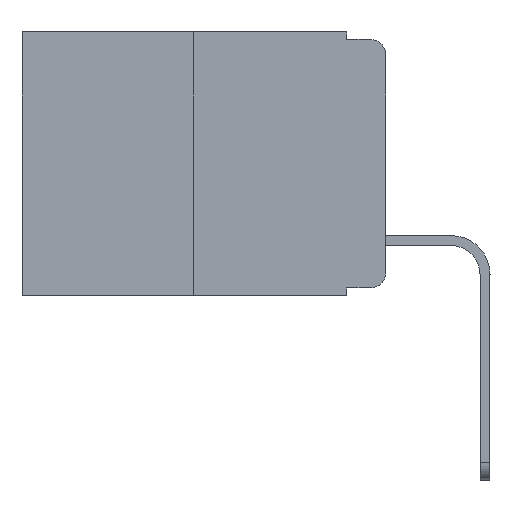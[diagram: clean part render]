
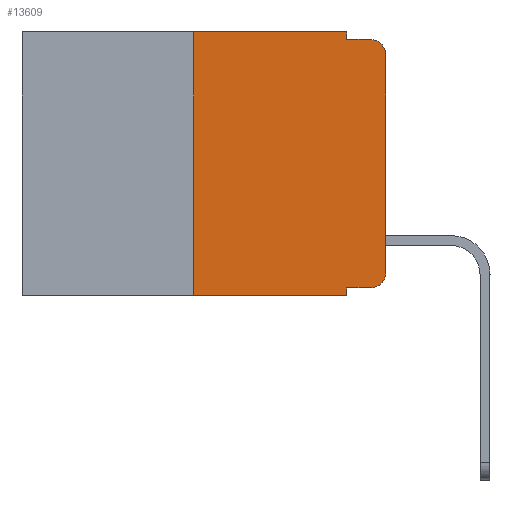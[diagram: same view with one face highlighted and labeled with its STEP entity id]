
A CAD part, left-side view. The second image highlights one B-rep face of the part: STEP entity #13609.
In plain terms, the highlighted planar face has unit normal (-1, 0, 0).
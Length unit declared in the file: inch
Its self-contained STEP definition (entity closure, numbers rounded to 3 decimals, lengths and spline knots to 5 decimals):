
#47 = CARTESIAN_POINT ( 'NONE',  ( 0., 0.25, -0.343 ) ) ;
#64 = CARTESIAN_POINT ( 'NONE',  ( 0., 0.051, 0. ) ) ;
#409 = DIRECTION ( 'NONE',  ( 0., 0., -1. ) ) ;
#425 = CARTESIAN_POINT ( 'NONE',  ( 0., 0., -0.313 ) ) ;
#571 = CARTESIAN_POINT ( 'NONE',  ( 0., 0.051, 0. ) ) ;
#805 = ORIENTED_EDGE ( 'NONE', *, *, #11514, .F. ) ;
#902 = ORIENTED_EDGE ( 'NONE', *, *, #3886, .F. ) ;
#1090 = VECTOR ( 'NONE', #4679, 39.37008 ) ;
#1252 = CARTESIAN_POINT ( 'NONE',  ( 0., 0.473, -0.343 ) ) ;
#1326 = DIRECTION ( 'NONE',  ( -1., 0., 0. ) ) ;
#1520 = EDGE_CURVE ( 'NONE', #8111, #6026, #4271, .T. ) ;
#1595 = EDGE_CURVE ( 'NONE', #8111, #5407, #14626, .T. ) ;
#1687 = VERTEX_POINT ( 'NONE', #5878 ) ;
#1738 = EDGE_CURVE ( 'NONE', #6319, #5173, #14802, .T. ) ;
#2243 = EDGE_CURVE ( 'NONE', #6086, #14339, #12147, .T. ) ;
#2329 = PLANE ( 'NONE',  #9129 ) ;
#3164 = CARTESIAN_POINT ( 'NONE',  ( 0., 0.02, -0.333 ) ) ;
#3420 = EDGE_CURVE ( 'NONE', #1687, #6319, #4641, .T. ) ;
#3616 = DIRECTION ( 'NONE',  ( 0., 0., -1. ) ) ;
#3622 = VERTEX_POINT ( 'NONE', #12099 ) ;
#3840 = EDGE_CURVE ( 'NONE', #3622, #13777, #6791, .T. ) ;
#3886 = EDGE_CURVE ( 'NONE', #1687, #6026, #6254, .T. ) ;
#4117 = ORIENTED_EDGE ( 'NONE', *, *, #14373, .T. ) ;
#4271 = LINE ( 'NONE', #1252, #13584 ) ;
#4641 = LINE ( 'NONE', #10659, #7683 ) ;
#4679 = DIRECTION ( 'NONE',  ( 0., -1., 0. ) ) ;
#5173 = VERTEX_POINT ( 'NONE', #425 ) ;
#5222 = CARTESIAN_POINT ( 'NONE',  ( 0., 0., 0. ) ) ;
#5407 = VERTEX_POINT ( 'NONE', #14429 ) ;
#5878 = CARTESIAN_POINT ( 'NONE',  ( 0., 0.051, -0.333 ) ) ;
#5891 = VECTOR ( 'NONE', #8561, 39.37008 ) ;
#6026 = VERTEX_POINT ( 'NONE', #13424 ) ;
#6086 = VERTEX_POINT ( 'NONE', #7729 ) ;
#6179 = EDGE_LOOP ( 'NONE', ( #4117, #11406, #805, #11504, #7063, #6339, #13868, #902, #12164, #9971 ) ) ;
#6184 = VECTOR ( 'NONE', #10897, 39.37008 ) ;
#6254 = LINE ( 'NONE', #64, #6424 ) ;
#6319 = VERTEX_POINT ( 'NONE', #3164 ) ;
#6339 = ORIENTED_EDGE ( 'NONE', *, *, #1595, .F. ) ;
#6424 = VECTOR ( 'NONE', #8051, 39.37008 ) ;
#6791 = CIRCLE ( 'NONE', #14113, 0.02 ) ;
#7063 = ORIENTED_EDGE ( 'NONE', *, *, #10193, .F. ) ;
#7683 = VECTOR ( 'NONE', #10703, 39.37008 ) ;
#7729 = CARTESIAN_POINT ( 'NONE',  ( 0., 0.051, 0. ) ) ;
#8051 = DIRECTION ( 'NONE',  ( 0., 0., -1. ) ) ;
#8089 = CARTESIAN_POINT ( 'NONE',  ( 0., 0.473, 0. ) ) ;
#8111 = VERTEX_POINT ( 'NONE', #47 ) ;
#8250 = DIRECTION ( 'NONE',  ( 0., 0., -1. ) ) ;
#8561 = DIRECTION ( 'NONE',  ( 0., 0., -1. ) ) ;
#8996 = LINE ( 'NONE', #11500, #1090 ) ;
#9129 = AXIS2_PLACEMENT_3D ( 'NONE', #8089, #9260, #3616 ) ;
#9260 = DIRECTION ( 'NONE',  ( 1., 0., 0. ) ) ;
#9635 = CARTESIAN_POINT ( 'NONE',  ( 0., 0.02, -0.01 ) ) ;
#9728 = AXIS2_PLACEMENT_3D ( 'NONE', #11967, #1326, #409 ) ;
#9971 = ORIENTED_EDGE ( 'NONE', *, *, #1738, .T. ) ;
#10193 = EDGE_CURVE ( 'NONE', #5407, #6086, #8996, .T. ) ;
#10221 = DIRECTION ( 'NONE',  ( 0., -1., 0. ) ) ;
#10350 = DIRECTION ( 'NONE',  ( -1., 0., 0. ) ) ;
#10493 = CARTESIAN_POINT ( 'NONE',  ( 0., 0.02, -0.03 ) ) ;
#10528 = DIRECTION ( 'NONE',  ( 0., 0., 1. ) ) ;
#10538 = VECTOR ( 'NONE', #10528, 39.37008 ) ;
#10659 = CARTESIAN_POINT ( 'NONE',  ( 0., 0.051, -0.333 ) ) ;
#10668 = LINE ( 'NONE', #5222, #6184 ) ;
#10703 = DIRECTION ( 'NONE',  ( 0., -1., 0. ) ) ;
#10709 = CARTESIAN_POINT ( 'NONE',  ( 0., 0.051, -0.01 ) ) ;
#10897 = DIRECTION ( 'NONE',  ( 0., 0., 1. ) ) ;
#11219 = FACE_OUTER_BOUND ( 'NONE', #6179, .T. ) ;
#11406 = ORIENTED_EDGE ( 'NONE', *, *, #3840, .T. ) ;
#11500 = CARTESIAN_POINT ( 'NONE',  ( 0., 0.473, 0. ) ) ;
#11504 = ORIENTED_EDGE ( 'NONE', *, *, #2243, .F. ) ;
#11514 = EDGE_CURVE ( 'NONE', #14339, #13777, #11787, .T. ) ;
#11787 = LINE ( 'NONE', #10709, #11974 ) ;
#11853 = DIRECTION ( 'NONE',  ( 0., -1., 0. ) ) ;
#11967 = CARTESIAN_POINT ( 'NONE',  ( 0., 0.02, -0.313 ) ) ;
#11974 = VECTOR ( 'NONE', #11853, 39.37008 ) ;
#12099 = CARTESIAN_POINT ( 'NONE',  ( 0., 0., -0.03 ) ) ;
#12147 = LINE ( 'NONE', #571, #5891 ) ;
#12164 = ORIENTED_EDGE ( 'NONE', *, *, #3420, .T. ) ;
#12884 = CARTESIAN_POINT ( 'NONE',  ( 0., 0.25, 0. ) ) ;
#13246 = CARTESIAN_POINT ( 'NONE',  ( 0., 0.051, -0.01 ) ) ;
#13424 = CARTESIAN_POINT ( 'NONE',  ( 0., 0.051, -0.343 ) ) ;
#13584 = VECTOR ( 'NONE', #10221, 39.37008 ) ;
#13609 = ADVANCED_FACE ( 'NONE', ( #11219 ), #2329, .F. ) ;
#13777 = VERTEX_POINT ( 'NONE', #9635 ) ;
#13868 = ORIENTED_EDGE ( 'NONE', *, *, #1520, .T. ) ;
#14113 = AXIS2_PLACEMENT_3D ( 'NONE', #10493, #10350, #8250 ) ;
#14339 = VERTEX_POINT ( 'NONE', #13246 ) ;
#14373 = EDGE_CURVE ( 'NONE', #5173, #3622, #10668, .T. ) ;
#14429 = CARTESIAN_POINT ( 'NONE',  ( 0., 0.25, 0. ) ) ;
#14626 = LINE ( 'NONE', #12884, #10538 ) ;
#14802 = CIRCLE ( 'NONE', #9728, 0.02 ) ;
